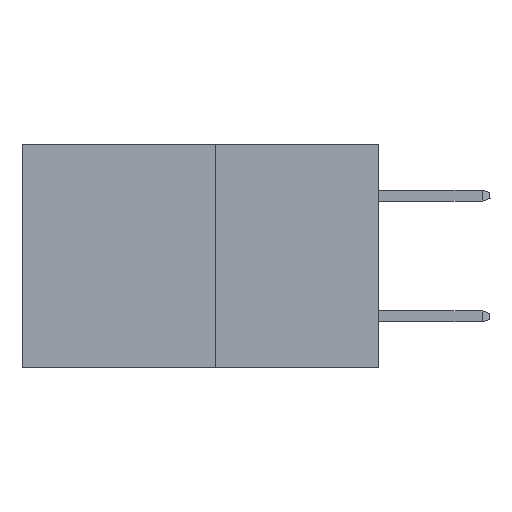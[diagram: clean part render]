
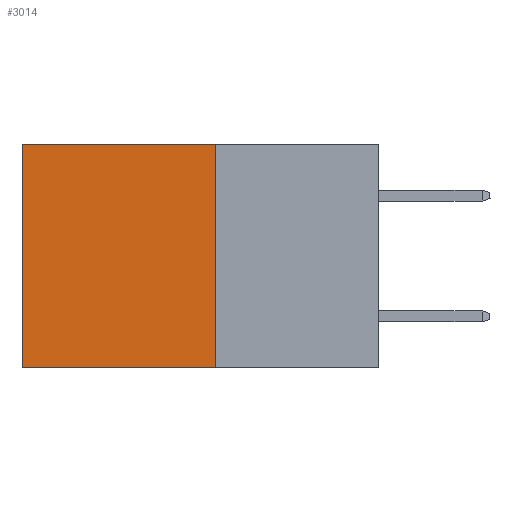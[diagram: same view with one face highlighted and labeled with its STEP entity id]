
A CAD part, left-side view. The second image highlights one B-rep face of the part: STEP entity #3014.
In plain terms, the highlighted planar face has unit normal (-1, 0, 0).
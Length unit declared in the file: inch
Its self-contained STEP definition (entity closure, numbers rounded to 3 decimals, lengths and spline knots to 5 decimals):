
#22 = DIRECTION ( 'NONE',  ( 0., 0., -1. ) ) ;
#52 = EDGE_LOOP ( 'NONE', ( #6178, #2939, #7919, #6540 ) ) ;
#480 = LINE ( 'NONE', #7563, #2208 ) ;
#646 = VERTEX_POINT ( 'NONE', #7043 ) ;
#692 = CARTESIAN_POINT ( 'NONE',  ( 0.277, 0.59, -0.37 ) ) ;
#1136 = CARTESIAN_POINT ( 'NONE',  ( 0.277, 0.59, 0. ) ) ;
#1838 = CARTESIAN_POINT ( 'NONE',  ( 0.277, 0.27, -0.37 ) ) ;
#2182 = EDGE_CURVE ( 'NONE', #646, #5930, #480, .T. ) ;
#2208 = VECTOR ( 'NONE', #7724, 39.37008 ) ;
#2447 = CARTESIAN_POINT ( 'NONE',  ( 0.277, 0.27, -0.37 ) ) ;
#2531 = VERTEX_POINT ( 'NONE', #6244 ) ;
#2566 = DIRECTION ( 'NONE',  ( 0., 1., 0. ) ) ;
#2939 = ORIENTED_EDGE ( 'NONE', *, *, #4989, .F. ) ;
#3014 = ADVANCED_FACE ( 'NONE', ( #4776 ), #5911, .F. ) ;
#3267 = VERTEX_POINT ( 'NONE', #692 ) ;
#3735 = LINE ( 'NONE', #4710, #6792 ) ;
#3836 = AXIS2_PLACEMENT_3D ( 'NONE', #2447, #6728, #22 ) ;
#4017 = DIRECTION ( 'NONE',  ( 0., 0., -1. ) ) ;
#4710 = CARTESIAN_POINT ( 'NONE',  ( 0.277, 0.27, -0.37 ) ) ;
#4776 = FACE_OUTER_BOUND ( 'NONE', #52, .T. ) ;
#4989 = EDGE_CURVE ( 'NONE', #2531, #3267, #6854, .T. ) ;
#5237 = CARTESIAN_POINT ( 'NONE',  ( 0.277, 0.59, -0.37 ) ) ;
#5301 = DIRECTION ( 'NONE',  ( 0., 0., -1. ) ) ;
#5911 = PLANE ( 'NONE',  #3836 ) ;
#5930 = VERTEX_POINT ( 'NONE', #1136 ) ;
#5945 = EDGE_CURVE ( 'NONE', #646, #2531, #3735, .T. ) ;
#6178 = ORIENTED_EDGE ( 'NONE', *, *, #7786, .T. ) ;
#6244 = CARTESIAN_POINT ( 'NONE',  ( 0.277, 0.27, -0.37 ) ) ;
#6540 = ORIENTED_EDGE ( 'NONE', *, *, #2182, .T. ) ;
#6678 = VECTOR ( 'NONE', #4017, 39.37008 ) ;
#6685 = VECTOR ( 'NONE', #2566, 39.37008 ) ;
#6728 = DIRECTION ( 'NONE',  ( 1., 0., 0. ) ) ;
#6792 = VECTOR ( 'NONE', #5301, 39.37008 ) ;
#6854 = LINE ( 'NONE', #1838, #6685 ) ;
#7043 = CARTESIAN_POINT ( 'NONE',  ( 0.277, 0.27, 0. ) ) ;
#7563 = CARTESIAN_POINT ( 'NONE',  ( 0.277, 0.27, 0. ) ) ;
#7724 = DIRECTION ( 'NONE',  ( 0., 1., 0. ) ) ;
#7786 = EDGE_CURVE ( 'NONE', #5930, #3267, #8219, .T. ) ;
#7919 = ORIENTED_EDGE ( 'NONE', *, *, #5945, .F. ) ;
#8219 = LINE ( 'NONE', #5237, #6678 ) ;
